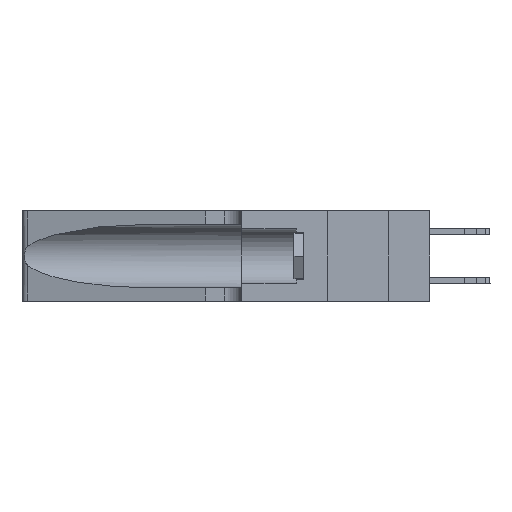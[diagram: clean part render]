
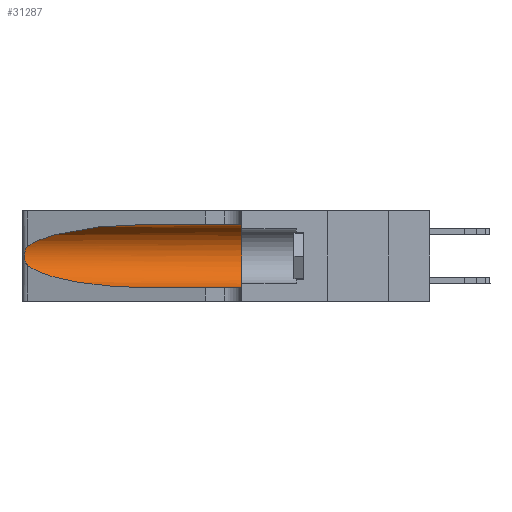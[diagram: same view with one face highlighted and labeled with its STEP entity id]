
A CAD part, left-side view. The second image highlights one B-rep face of the part: STEP entity #31287.
In plain terms, the highlighted cylindrical face has radius 3.308 mm (diameter 6.617 mm), a partial arc.
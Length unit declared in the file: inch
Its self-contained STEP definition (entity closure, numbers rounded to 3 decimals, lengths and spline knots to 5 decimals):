
#28 = EDGE_CURVE ( 'NONE', #11197, #23948, #6326, .T. ) ;
#378 = CARTESIAN_POINT ( 'NONE',  ( 0.25789, 1.23486, 0.15765 ) ) ;
#1245 = CARTESIAN_POINT ( 'NONE',  ( 0.25487, 1.22718, 0.22369 ) ) ;
#1685 = CARTESIAN_POINT ( 'NONE',  ( 0.1305, 0.72297, 0.31525 ) ) ;
#1848 = EDGE_LOOP ( 'NONE', ( #8084, #30010, #3744, #21463, #3140, #5355 ) ) ;
#1906 = CARTESIAN_POINT ( 'NONE',  ( 0.1305, 0.72297, 0.05475 ) ) ;
#2265 = CARTESIAN_POINT ( 'NONE',  ( 0.1305, 1.61858, 0.31525 ) ) ;
#2621 = DIRECTION ( 'NONE',  ( 0., -1., 0. ) ) ;
#3140 = ORIENTED_EDGE ( 'NONE', *, *, #29929, .F. ) ;
#3218 = AXIS2_PLACEMENT_3D ( 'NONE', #13152, #12736, #8033 ) ;
#3744 = ORIENTED_EDGE ( 'NONE', *, *, #28, .T. ) ;
#3889 = CARTESIAN_POINT ( 'NONE',  ( 0.1305, 0.72297, 0.05475 ) ) ;
#4042 = EDGE_CURVE ( 'NONE', #21008, #11197, #30299, .T. ) ;
#4250 = CARTESIAN_POINT ( 'NONE',  ( 0.26018, 1.23835, 0.19895 ) ) ;
#4466 = LINE ( 'NONE', #30681, #25746 ) ;
#5355 = ORIENTED_EDGE ( 'NONE', *, *, #16502, .F. ) ;
#6004 = CARTESIAN_POINT ( 'NONE',  ( 0.25555, 1.22994, 0.2215 ) ) ;
#6253 = CARTESIAN_POINT ( 'NONE',  ( 0.25487, 1.22718, 0.14631 ) ) ;
#6326 =( BOUNDED_CURVE ( )  B_SPLINE_CURVE ( 3, ( #7245, #7350, #32473, #1906 ),
 .UNSPECIFIED., .F., .F. ) 
 B_SPLINE_CURVE_WITH_KNOTS ( ( 4, 4 ),
 ( 3.44316, 4.71239 ),
 .UNSPECIFIED. ) 
 CURVE ( )  GEOMETRIC_REPRESENTATION_ITEM ( )  RATIONAL_B_SPLINE_CURVE ( ( 1., 0.87, 0.87, 1. ) ) 
 REPRESENTATION_ITEM ( '' )  );
#6817 = CARTESIAN_POINT ( 'NONE',  ( 0.25487, 1.22718, 0.22369 ) ) ;
#7040 = CARTESIAN_POINT ( 'NONE',  ( 0.25856, 1.23593, 0.16098 ) ) ;
#7245 = CARTESIAN_POINT ( 'NONE',  ( 0.25487, 1.22718, 0.14631 ) ) ;
#7350 = CARTESIAN_POINT ( 'NONE',  ( 0.2373, 1.15595, 0.08982 ) ) ;
#8033 = DIRECTION ( 'NONE',  ( 0., 0., 1. ) ) ;
#8084 = ORIENTED_EDGE ( 'NONE', *, *, #19006, .T. ) ;
#8552 = FACE_OUTER_BOUND ( 'NONE', #1848, .T. ) ;
#8845 = CARTESIAN_POINT ( 'NONE',  ( 0.25639, 1.23184, 0.21858 ) ) ;
#9348 = CARTESIAN_POINT ( 'NONE',  ( 0.26075, 1.23896, 0.19203 ) ) ;
#9459 = CARTESIAN_POINT ( 'NONE',  ( 0.26017, 1.23833, 0.17102 ) ) ;
#9547 = CARTESIAN_POINT ( 'NONE',  ( 0.18966, 0.96281, 0.31525 ) ) ;
#10722 = VERTEX_POINT ( 'NONE', #21921 ) ;
#11197 = VERTEX_POINT ( 'NONE', #6253 ) ;
#12736 = DIRECTION ( 'NONE',  ( 0., 1., 0. ) ) ;
#13152 = CARTESIAN_POINT ( 'NONE',  ( 0.1305, 0.35, 0.185 ) ) ;
#14510 = CARTESIAN_POINT ( 'NONE',  ( 0.25854, 1.2359, 0.20912 ) ) ;
#15401 = CARTESIAN_POINT ( 'NONE',  ( 0.1305, 1.61858, 0.185 ) ) ;
#16060 = CARTESIAN_POINT ( 'NONE',  ( 0.1305, 0.35, 0.31525 ) ) ;
#16502 = EDGE_CURVE ( 'NONE', #16803, #22407, #20998, .T. ) ;
#16803 = VERTEX_POINT ( 'NONE', #1685 ) ;
#17001 = CARTESIAN_POINT ( 'NONE',  ( 0.1305, 0.72297, 0.31525 ) ) ;
#19006 = EDGE_CURVE ( 'NONE', #16803, #21008, #20463, .T. ) ;
#19673 = CARTESIAN_POINT ( 'NONE',  ( 0.25555, 1.22993, 0.14849 ) ) ;
#20017 = DIRECTION ( 'NONE',  ( 0., -1., 0. ) ) ;
#20147 = DIRECTION ( 'NONE',  ( 0., 0., -1. ) ) ;
#20463 =( BOUNDED_CURVE ( )  B_SPLINE_CURVE ( 3, ( #17001, #9547, #21977, #26908 ),
 .UNSPECIFIED., .F., .T. ) 
 B_SPLINE_CURVE_WITH_KNOTS ( ( 4, 4 ),
 ( 1.5708, 2.84003 ),
 .UNSPECIFIED. ) 
 CURVE ( )  GEOMETRIC_REPRESENTATION_ITEM ( )  RATIONAL_B_SPLINE_CURVE ( ( 1., 0.87, 0.87, 1. ) ) 
 REPRESENTATION_ITEM ( '' )  );
#20593 = DIRECTION ( 'NONE',  ( 0., -1., 0. ) ) ;
#20998 = LINE ( 'NONE', #2265, #22628 ) ;
#21008 = VERTEX_POINT ( 'NONE', #1245 ) ;
#21463 = ORIENTED_EDGE ( 'NONE', *, *, #32455, .T. ) ;
#21921 = CARTESIAN_POINT ( 'NONE',  ( 0.1305, 0.35, 0.05475 ) ) ;
#21977 = CARTESIAN_POINT ( 'NONE',  ( 0.2373, 1.15595, 0.28018 ) ) ;
#22407 = VERTEX_POINT ( 'NONE', #16060 ) ;
#22628 = VECTOR ( 'NONE', #20017, 39.37008 ) ;
#23948 = VERTEX_POINT ( 'NONE', #3889 ) ;
#24300 = CARTESIAN_POINT ( 'NONE',  ( 0.25787, 1.23484, 0.2124 ) ) ;
#24518 = CARTESIAN_POINT ( 'NONE',  ( 0.26075, 1.23896, 0.178 ) ) ;
#25746 = VECTOR ( 'NONE', #20593, 39.37008 ) ;
#25899 = AXIS2_PLACEMENT_3D ( 'NONE', #15401, #2621, #20147 ) ;
#25915 = CARTESIAN_POINT ( 'NONE',  ( 0.25487, 1.22718, 0.14631 ) ) ;
#26908 = CARTESIAN_POINT ( 'NONE',  ( 0.25487, 1.22718, 0.22369 ) ) ;
#27424 = CYLINDRICAL_SURFACE ( 'NONE', #25899, 0.13025 ) ;
#27516 = CIRCLE ( 'NONE', #3218, 0.13025 ) ;
#29929 = EDGE_CURVE ( 'NONE', #22407, #10722, #27516, .T. ) ;
#30010 = ORIENTED_EDGE ( 'NONE', *, *, #4042, .T. ) ;
#30299 = B_SPLINE_CURVE_WITH_KNOTS ( 'NONE', 3,
 ( #6817, #6004, #8845, #24300, #14510, #4250, #9348, #24518, #9459, #7040, #378, #30639, #19673, #25915 ),
 .UNSPECIFIED., .F., .F.,
 ( 4, 2, 2, 2, 2, 2, 4 ),
 ( 0., 0.00027, 0.00053, 0.00107, 0.0016, 0.00187, 0.00214 ),
 .UNSPECIFIED. ) ;
#30639 = CARTESIAN_POINT ( 'NONE',  ( 0.25639, 1.23186, 0.15144 ) ) ;
#30681 = CARTESIAN_POINT ( 'NONE',  ( 0.1305, 1.61858, 0.05475 ) ) ;
#31287 = ADVANCED_FACE ( 'NONE', ( #8552 ), #27424, .F. ) ;
#32455 = EDGE_CURVE ( 'NONE', #23948, #10722, #4466, .T. ) ;
#32473 = CARTESIAN_POINT ( 'NONE',  ( 0.18966, 0.96281, 0.05475 ) ) ;
